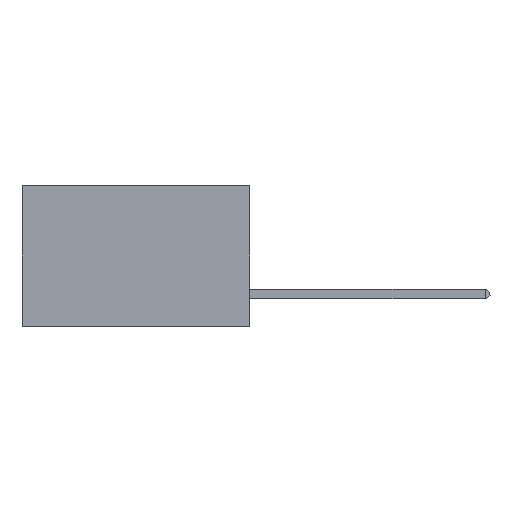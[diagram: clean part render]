
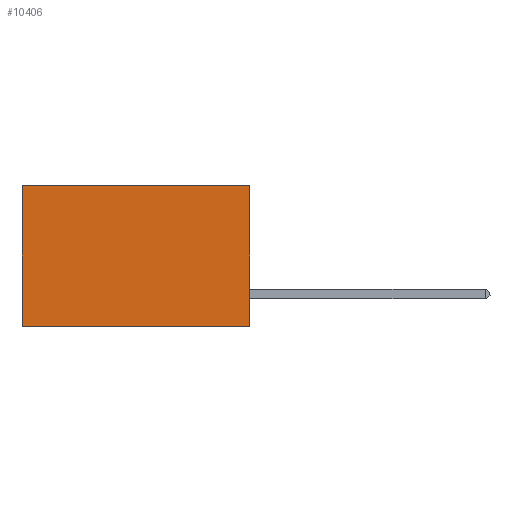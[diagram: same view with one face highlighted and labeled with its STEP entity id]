
A CAD part, left-side view. The second image highlights one B-rep face of the part: STEP entity #10406.
In plain terms, the highlighted planar face has unit normal (-1, 0, 0).
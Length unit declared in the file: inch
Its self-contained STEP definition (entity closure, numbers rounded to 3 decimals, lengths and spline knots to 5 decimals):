
#792 = CARTESIAN_POINT ( 'NONE',  ( 0.2875, 0., 0. ) ) ;
#1582 = LINE ( 'NONE', #10844, #12587 ) ;
#1656 = VECTOR ( 'NONE', #13714, 39.37008 ) ;
#1893 = FACE_OUTER_BOUND ( 'NONE', #16473, .T. ) ;
#2399 = ORIENTED_EDGE ( 'NONE', *, *, #5323, .T. ) ;
#3204 = AXIS2_PLACEMENT_3D ( 'NONE', #15161, #7574, #8618 ) ;
#3322 = LINE ( 'NONE', #7128, #4323 ) ;
#3632 = DIRECTION ( 'NONE',  ( 0., 0., -1. ) ) ;
#3821 = CARTESIAN_POINT ( 'NONE',  ( 0.2875, 0.6, -0.37 ) ) ;
#4323 = VECTOR ( 'NONE', #16074, 39.37008 ) ;
#4673 = CARTESIAN_POINT ( 'NONE',  ( 0.2875, 0.6, 0. ) ) ;
#4867 = CARTESIAN_POINT ( 'NONE',  ( 0.2875, 0., 0. ) ) ;
#5323 = EDGE_CURVE ( 'NONE', #8429, #15455, #6066, .T. ) ;
#5784 = DIRECTION ( 'NONE',  ( 0., 0., -1. ) ) ;
#5856 = VECTOR ( 'NONE', #3632, 39.37008 ) ;
#6066 = LINE ( 'NONE', #792, #1656 ) ;
#6558 = VERTEX_POINT ( 'NONE', #3821 ) ;
#6875 = VERTEX_POINT ( 'NONE', #7346 ) ;
#7128 = CARTESIAN_POINT ( 'NONE',  ( 0.2875, 0., -0.37 ) ) ;
#7346 = CARTESIAN_POINT ( 'NONE',  ( 0.2875, 0., -0.37 ) ) ;
#7372 = EDGE_CURVE ( 'NONE', #15455, #6558, #1582, .T. ) ;
#7574 = DIRECTION ( 'NONE',  ( 1., 0., 0. ) ) ;
#8429 = VERTEX_POINT ( 'NONE', #13120 ) ;
#8618 = DIRECTION ( 'NONE',  ( 0., 0., -1. ) ) ;
#9639 = ORIENTED_EDGE ( 'NONE', *, *, #14860, .F. ) ;
#9954 = PLANE ( 'NONE',  #3204 ) ;
#10406 = ADVANCED_FACE ( 'NONE', ( #1893 ), #9954, .F. ) ;
#10844 = CARTESIAN_POINT ( 'NONE',  ( 0.2875, 0.6, 0. ) ) ;
#12587 = VECTOR ( 'NONE', #5784, 39.37008 ) ;
#13120 = CARTESIAN_POINT ( 'NONE',  ( 0.2875, 0., 0. ) ) ;
#13714 = DIRECTION ( 'NONE',  ( 0., 1., 0. ) ) ;
#13824 = EDGE_CURVE ( 'NONE', #8429, #6875, #15371, .T. ) ;
#14173 = ORIENTED_EDGE ( 'NONE', *, *, #13824, .F. ) ;
#14307 = ORIENTED_EDGE ( 'NONE', *, *, #7372, .T. ) ;
#14860 = EDGE_CURVE ( 'NONE', #6875, #6558, #3322, .T. ) ;
#15161 = CARTESIAN_POINT ( 'NONE',  ( 0.2875, 0., 0. ) ) ;
#15371 = LINE ( 'NONE', #4867, #5856 ) ;
#15455 = VERTEX_POINT ( 'NONE', #4673 ) ;
#16074 = DIRECTION ( 'NONE',  ( 0., 1., 0. ) ) ;
#16473 = EDGE_LOOP ( 'NONE', ( #14307, #9639, #14173, #2399 ) ) ;
